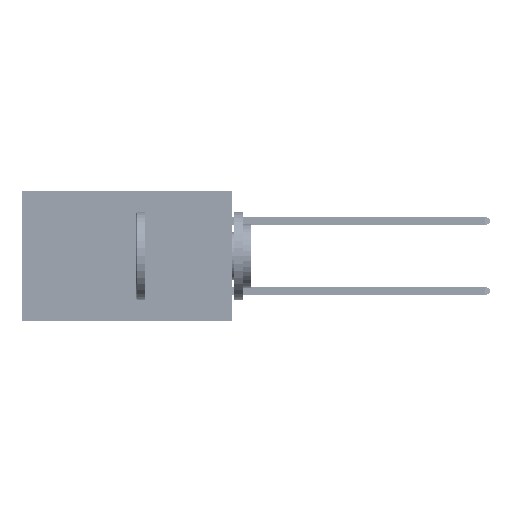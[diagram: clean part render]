
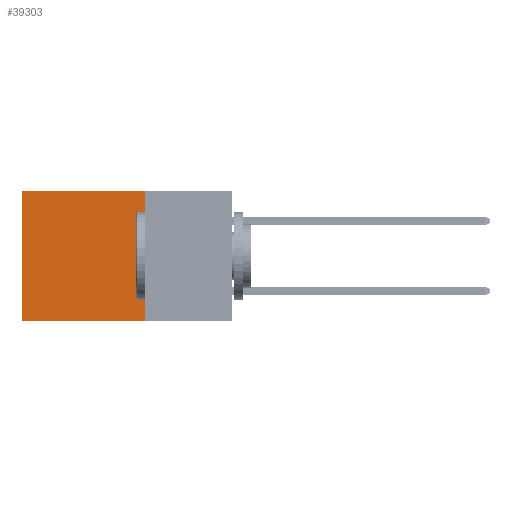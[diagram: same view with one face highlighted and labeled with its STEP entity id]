
A CAD part, left-side view. The second image highlights one B-rep face of the part: STEP entity #39303.
In plain terms, the highlighted planar face has unit normal (-1, 0, 0).
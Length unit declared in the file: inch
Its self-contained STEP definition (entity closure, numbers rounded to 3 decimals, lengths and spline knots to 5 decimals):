
#584 = CARTESIAN_POINT ( 'NONE',  ( 0.2875, 0.6, 0. ) ) ;
#1262 = ORIENTED_EDGE ( 'NONE', *, *, #24581, .T. ) ;
#3551 = ORIENTED_EDGE ( 'NONE', *, *, #23452, .F. ) ;
#5517 = VECTOR ( 'NONE', #46378, 39.37008 ) ;
#6000 = PLANE ( 'NONE',  #16784 ) ;
#6117 = DIRECTION ( 'NONE',  ( 0., 1., 0. ) ) ;
#6189 = CARTESIAN_POINT ( 'NONE',  ( 0.2875, 0.25, -0.37 ) ) ;
#6276 = VECTOR ( 'NONE', #11728, 39.37008 ) ;
#6725 = LINE ( 'NONE', #584, #5517 ) ;
#11728 = DIRECTION ( 'NONE',  ( 0., 0., -1. ) ) ;
#16784 = AXIS2_PLACEMENT_3D ( 'NONE', #17610, #25981, #37015 ) ;
#17610 = CARTESIAN_POINT ( 'NONE',  ( 0.2875, 0.25, 0. ) ) ;
#19604 = VECTOR ( 'NONE', #32719, 39.37008 ) ;
#19785 = CARTESIAN_POINT ( 'NONE',  ( 0.2875, 0.6, 0. ) ) ;
#20637 = EDGE_CURVE ( 'NONE', #47004, #33527, #28556, .T. ) ;
#20688 = CARTESIAN_POINT ( 'NONE',  ( 0.2875, 0.25, 0. ) ) ;
#21165 = VERTEX_POINT ( 'NONE', #19785 ) ;
#21493 = CARTESIAN_POINT ( 'NONE',  ( 0.2875, 0.6, -0.37 ) ) ;
#22766 = LINE ( 'NONE', #48256, #31111 ) ;
#23197 = LINE ( 'NONE', #20688, #19604 ) ;
#23452 = EDGE_CURVE ( 'NONE', #33527, #39355, #22766, .T. ) ;
#23945 = EDGE_LOOP ( 'NONE', ( #44351, #3551, #37644, #1262 ) ) ;
#24581 = EDGE_CURVE ( 'NONE', #47004, #21165, #23197, .T. ) ;
#25981 = DIRECTION ( 'NONE',  ( 1., 0., 0. ) ) ;
#26866 = EDGE_CURVE ( 'NONE', #21165, #39355, #6725, .T. ) ;
#28556 = LINE ( 'NONE', #42090, #6276 ) ;
#31111 = VECTOR ( 'NONE', #6117, 39.37008 ) ;
#32719 = DIRECTION ( 'NONE',  ( 0., 1., 0. ) ) ;
#33527 = VERTEX_POINT ( 'NONE', #6189 ) ;
#37015 = DIRECTION ( 'NONE',  ( 0., 0., -1. ) ) ;
#37644 = ORIENTED_EDGE ( 'NONE', *, *, #20637, .F. ) ;
#37895 = CARTESIAN_POINT ( 'NONE',  ( 0.2875, 0.25, 0. ) ) ;
#39303 = ADVANCED_FACE ( 'NONE', ( #40235 ), #6000, .F. ) ;
#39355 = VERTEX_POINT ( 'NONE', #21493 ) ;
#40235 = FACE_OUTER_BOUND ( 'NONE', #23945, .T. ) ;
#42090 = CARTESIAN_POINT ( 'NONE',  ( 0.2875, 0.25, 0. ) ) ;
#44351 = ORIENTED_EDGE ( 'NONE', *, *, #26866, .T. ) ;
#46378 = DIRECTION ( 'NONE',  ( 0., 0., -1. ) ) ;
#47004 = VERTEX_POINT ( 'NONE', #37895 ) ;
#48256 = CARTESIAN_POINT ( 'NONE',  ( 0.2875, 0.25, -0.37 ) ) ;
